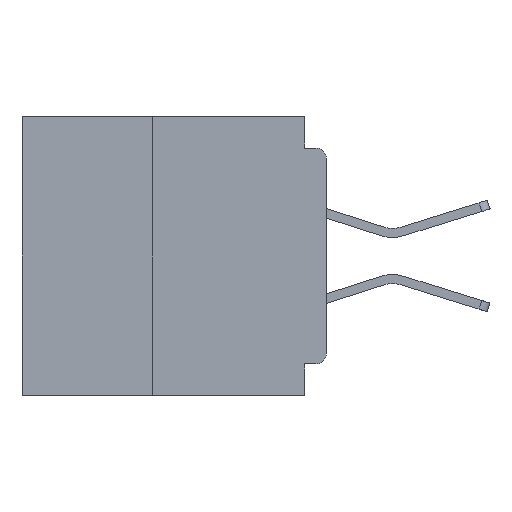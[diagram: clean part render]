
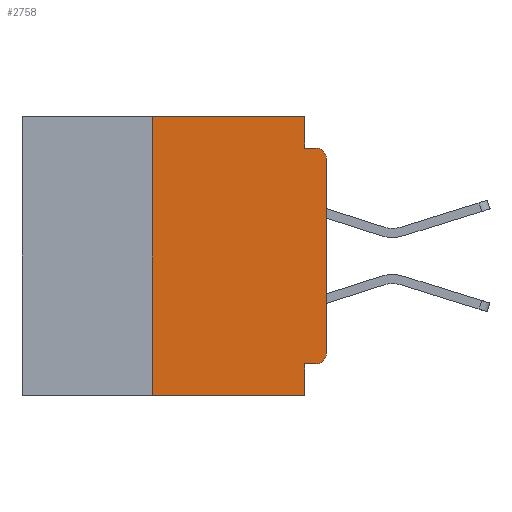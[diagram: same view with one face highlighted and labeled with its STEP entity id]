
A CAD part, left-side view. The second image highlights one B-rep face of the part: STEP entity #2758.
In plain terms, the highlighted planar face has unit normal (-1, 0, 0).
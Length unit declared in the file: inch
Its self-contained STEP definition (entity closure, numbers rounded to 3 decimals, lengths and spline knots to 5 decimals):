
#420 = PLANE ( 'NONE',  #38288 ) ;
#997 = EDGE_CURVE ( 'NONE', #18003, #2837, #31608, .T. ) ;
#1674 = DIRECTION ( 'NONE',  ( 0., 0., -1. ) ) ;
#2063 = ORIENTED_EDGE ( 'NONE', *, *, #38408, .T. ) ;
#2094 = ORIENTED_EDGE ( 'NONE', *, *, #20493, .T. ) ;
#2758 = ADVANCED_FACE ( 'NONE', ( #14104 ), #420, .F. ) ;
#2837 = VERTEX_POINT ( 'NONE', #16816 ) ;
#3722 = DIRECTION ( 'NONE',  ( 0., 0., -1. ) ) ;
#3808 = CARTESIAN_POINT ( 'NONE',  ( 0., 0., -0.34 ) ) ;
#4546 = DIRECTION ( 'NONE',  ( 0., -1., 0. ) ) ;
#4670 = LINE ( 'NONE', #35287, #18732 ) ;
#4979 = CARTESIAN_POINT ( 'NONE',  ( 0., 0.031, -0.045 ) ) ;
#5015 = CARTESIAN_POINT ( 'NONE',  ( 0., 0.015, -0.355 ) ) ;
#5023 = AXIS2_PLACEMENT_3D ( 'NONE', #7885, #30242, #11130 ) ;
#5880 = AXIS2_PLACEMENT_3D ( 'NONE', #28173, #8998, #31351 ) ;
#6125 = ORIENTED_EDGE ( 'NONE', *, *, #7023, .T. ) ;
#6456 = VERTEX_POINT ( 'NONE', #4979 ) ;
#6742 = VECTOR ( 'NONE', #28047, 39.37008 ) ;
#7023 = EDGE_CURVE ( 'NONE', #27042, #13954, #7077, .T. ) ;
#7077 = CIRCLE ( 'NONE', #5023, 0.015 ) ;
#7617 = CARTESIAN_POINT ( 'NONE',  ( 0., 0., -0.045 ) ) ;
#7785 = VERTEX_POINT ( 'NONE', #5015 ) ;
#7885 = CARTESIAN_POINT ( 'NONE',  ( 0., 0.015, -0.06 ) ) ;
#8379 = CARTESIAN_POINT ( 'NONE',  ( 0., 0.437, -0.4 ) ) ;
#8934 = EDGE_LOOP ( 'NONE', ( #2063, #6125, #30329, #12570, #39807, #10969, #2094, #20709, #12353, #15207 ) ) ;
#8998 = DIRECTION ( 'NONE',  ( -1., 0., 0. ) ) ;
#10174 = LINE ( 'NONE', #7617, #32618 ) ;
#10969 = ORIENTED_EDGE ( 'NONE', *, *, #997, .F. ) ;
#10970 = VECTOR ( 'NONE', #30425, 39.37008 ) ;
#11130 = DIRECTION ( 'NONE',  ( 0., 0., -1. ) ) ;
#11157 = VECTOR ( 'NONE', #18851, 39.37008 ) ;
#11778 = CIRCLE ( 'NONE', #5880, 0.015 ) ;
#11991 = CARTESIAN_POINT ( 'NONE',  ( 0., 0.437, 0. ) ) ;
#12353 = ORIENTED_EDGE ( 'NONE', *, *, #26888, .F. ) ;
#12570 = ORIENTED_EDGE ( 'NONE', *, *, #19049, .F. ) ;
#13190 = LINE ( 'NONE', #15661, #11157 ) ;
#13954 = VERTEX_POINT ( 'NONE', #39446 ) ;
#14104 = FACE_OUTER_BOUND ( 'NONE', #8934, .T. ) ;
#15207 = ORIENTED_EDGE ( 'NONE', *, *, #37691, .T. ) ;
#15358 = EDGE_CURVE ( 'NONE', #2837, #22792, #40067, .T. ) ;
#15661 = CARTESIAN_POINT ( 'NONE',  ( 0., 0., -0.355 ) ) ;
#16284 = VERTEX_POINT ( 'NONE', #35561 ) ;
#16542 = CARTESIAN_POINT ( 'NONE',  ( 0., 0.437, 0. ) ) ;
#16768 = LINE ( 'NONE', #39911, #26224 ) ;
#16816 = CARTESIAN_POINT ( 'NONE',  ( 0., 0.25, 0. ) ) ;
#18003 = VERTEX_POINT ( 'NONE', #31480 ) ;
#18113 = DIRECTION ( 'NONE',  ( 0., -1., 0. ) ) ;
#18732 = VECTOR ( 'NONE', #19490, 39.37008 ) ;
#18851 = DIRECTION ( 'NONE',  ( 0., 1., 0. ) ) ;
#19049 = EDGE_CURVE ( 'NONE', #22792, #6456, #28958, .T. ) ;
#19160 = CARTESIAN_POINT ( 'NONE',  ( 0., 0.031, -0.355 ) ) ;
#19490 = DIRECTION ( 'NONE',  ( 0., 0., 1. ) ) ;
#20493 = EDGE_CURVE ( 'NONE', #18003, #16284, #36712, .T. ) ;
#20709 = ORIENTED_EDGE ( 'NONE', *, *, #33080, .F. ) ;
#21233 = VERTEX_POINT ( 'NONE', #19160 ) ;
#22792 = VERTEX_POINT ( 'NONE', #33309 ) ;
#26224 = VECTOR ( 'NONE', #1674, 39.37008 ) ;
#26570 = EDGE_CURVE ( 'NONE', #6456, #13954, #10174, .T. ) ;
#26888 = EDGE_CURVE ( 'NONE', #7785, #21233, #13190, .T. ) ;
#27042 = VERTEX_POINT ( 'NONE', #38363 ) ;
#28047 = DIRECTION ( 'NONE',  ( 0., -1., 0. ) ) ;
#28173 = CARTESIAN_POINT ( 'NONE',  ( 0., 0.015, -0.34 ) ) ;
#28314 = VECTOR ( 'NONE', #18113, 39.37008 ) ;
#28659 = VERTEX_POINT ( 'NONE', #3808 ) ;
#28958 = LINE ( 'NONE', #33453, #10970 ) ;
#30242 = DIRECTION ( 'NONE',  ( -1., 0., 0. ) ) ;
#30329 = ORIENTED_EDGE ( 'NONE', *, *, #26570, .F. ) ;
#30425 = DIRECTION ( 'NONE',  ( 0., 0., -1. ) ) ;
#31351 = DIRECTION ( 'NONE',  ( 0., 0., -1. ) ) ;
#31480 = CARTESIAN_POINT ( 'NONE',  ( 0., 0.25, -0.4 ) ) ;
#31608 = LINE ( 'NONE', #40981, #39997 ) ;
#32618 = VECTOR ( 'NONE', #4546, 39.37008 ) ;
#33080 = EDGE_CURVE ( 'NONE', #21233, #16284, #16768, .T. ) ;
#33309 = CARTESIAN_POINT ( 'NONE',  ( 0., 0.031, 0. ) ) ;
#33453 = CARTESIAN_POINT ( 'NONE',  ( 0., 0.031, 0. ) ) ;
#35287 = CARTESIAN_POINT ( 'NONE',  ( 0., 0., 0. ) ) ;
#35534 = DIRECTION ( 'NONE',  ( 1., 0., 0. ) ) ;
#35561 = CARTESIAN_POINT ( 'NONE',  ( 0., 0.031, -0.4 ) ) ;
#36712 = LINE ( 'NONE', #8379, #28314 ) ;
#37691 = EDGE_CURVE ( 'NONE', #7785, #28659, #11778, .T. ) ;
#38288 = AXIS2_PLACEMENT_3D ( 'NONE', #16542, #35534, #3722 ) ;
#38363 = CARTESIAN_POINT ( 'NONE',  ( 0., 0., -0.06 ) ) ;
#38408 = EDGE_CURVE ( 'NONE', #28659, #27042, #4670, .T. ) ;
#39446 = CARTESIAN_POINT ( 'NONE',  ( 0., 0.015, -0.045 ) ) ;
#39545 = DIRECTION ( 'NONE',  ( 0., 0., 1. ) ) ;
#39807 = ORIENTED_EDGE ( 'NONE', *, *, #15358, .F. ) ;
#39911 = CARTESIAN_POINT ( 'NONE',  ( 0., 0.031, -0.4 ) ) ;
#39997 = VECTOR ( 'NONE', #39545, 39.37008 ) ;
#40067 = LINE ( 'NONE', #11991, #6742 ) ;
#40981 = CARTESIAN_POINT ( 'NONE',  ( 0., 0.25, -0.4 ) ) ;
